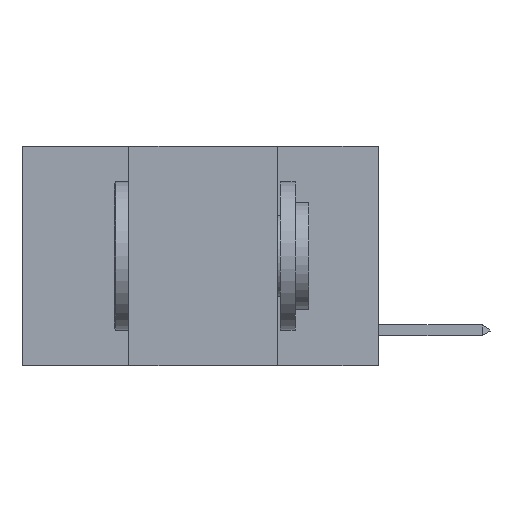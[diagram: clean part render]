
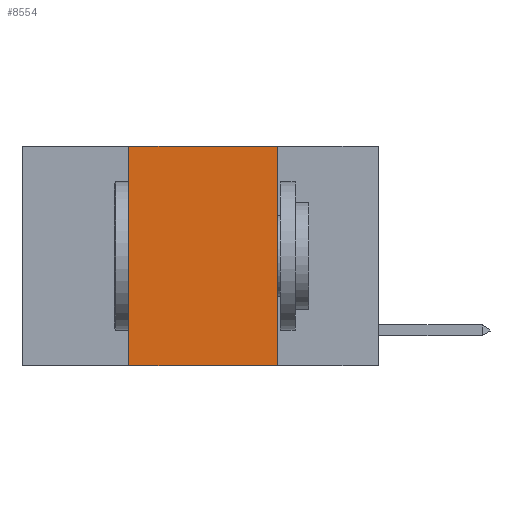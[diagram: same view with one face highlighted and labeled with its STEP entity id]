
A CAD part, left-side view. The second image highlights one B-rep face of the part: STEP entity #8554.
In plain terms, the highlighted planar face has unit normal (-1, 0, 0).
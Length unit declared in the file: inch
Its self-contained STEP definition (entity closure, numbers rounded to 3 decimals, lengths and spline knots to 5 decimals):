
#246 = CARTESIAN_POINT ( 'NONE',  ( 0., 0.42, -0.37 ) ) ;
#614 = CARTESIAN_POINT ( 'NONE',  ( 0., 0.6, 0. ) ) ;
#1960 = CARTESIAN_POINT ( 'NONE',  ( 0., 0.6, 0. ) ) ;
#2248 = DIRECTION ( 'NONE',  ( 0., -1., 0. ) ) ;
#2528 = EDGE_CURVE ( 'NONE', #7170, #8124, #3059, .T. ) ;
#2693 = PLANE ( 'NONE',  #7952 ) ;
#3059 = LINE ( 'NONE', #1960, #3400 ) ;
#3322 = VECTOR ( 'NONE', #3921, 39.37008 ) ;
#3400 = VECTOR ( 'NONE', #2248, 39.37008 ) ;
#3422 = ORIENTED_EDGE ( 'NONE', *, *, #2528, .F. ) ;
#3576 = ORIENTED_EDGE ( 'NONE', *, *, #8139, .F. ) ;
#3773 = DIRECTION ( 'NONE',  ( 1., 0., 0. ) ) ;
#3815 = VERTEX_POINT ( 'NONE', #246 ) ;
#3921 = DIRECTION ( 'NONE',  ( 0., 0., -1. ) ) ;
#4252 = DIRECTION ( 'NONE',  ( 0., 0., 1. ) ) ;
#5303 = LINE ( 'NONE', #10731, #7732 ) ;
#5432 = LINE ( 'NONE', #11451, #10890 ) ;
#5802 = FACE_OUTER_BOUND ( 'NONE', #8636, .T. ) ;
#6045 = CARTESIAN_POINT ( 'NONE',  ( 0., 0.17, 0. ) ) ;
#7170 = VERTEX_POINT ( 'NONE', #12663 ) ;
#7732 = VECTOR ( 'NONE', #12773, 39.37008 ) ;
#7952 = AXIS2_PLACEMENT_3D ( 'NONE', #614, #3773, #10998 ) ;
#8124 = VERTEX_POINT ( 'NONE', #11128 ) ;
#8134 = ORIENTED_EDGE ( 'NONE', *, *, #12035, .F. ) ;
#8139 = EDGE_CURVE ( 'NONE', #8124, #8218, #8535, .T. ) ;
#8218 = VERTEX_POINT ( 'NONE', #11259 ) ;
#8393 = EDGE_CURVE ( 'NONE', #3815, #8218, #5303, .T. ) ;
#8535 = LINE ( 'NONE', #6045, #3322 ) ;
#8554 = ADVANCED_FACE ( 'NONE', ( #5802 ), #2693, .F. ) ;
#8636 = EDGE_LOOP ( 'NONE', ( #3576, #3422, #8134, #11066 ) ) ;
#10731 = CARTESIAN_POINT ( 'NONE',  ( 0., 0.6, -0.37 ) ) ;
#10890 = VECTOR ( 'NONE', #4252, 39.37008 ) ;
#10998 = DIRECTION ( 'NONE',  ( 0., 0., -1. ) ) ;
#11066 = ORIENTED_EDGE ( 'NONE', *, *, #8393, .T. ) ;
#11128 = CARTESIAN_POINT ( 'NONE',  ( 0., 0.17, 0. ) ) ;
#11259 = CARTESIAN_POINT ( 'NONE',  ( 0., 0.17, -0.37 ) ) ;
#11451 = CARTESIAN_POINT ( 'NONE',  ( 0., 0.42, 0. ) ) ;
#12035 = EDGE_CURVE ( 'NONE', #3815, #7170, #5432, .T. ) ;
#12663 = CARTESIAN_POINT ( 'NONE',  ( 0., 0.42, 0. ) ) ;
#12773 = DIRECTION ( 'NONE',  ( 0., -1., 0. ) ) ;
